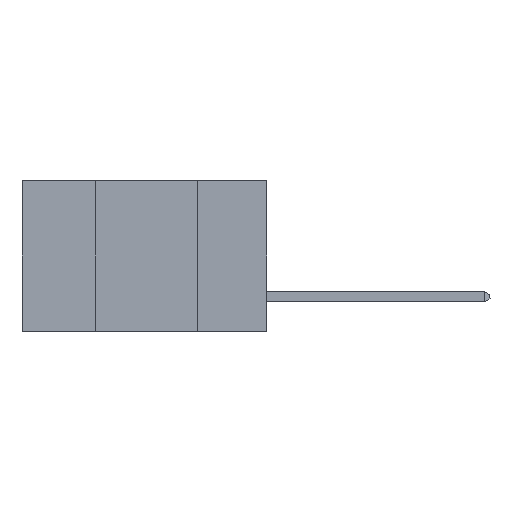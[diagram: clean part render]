
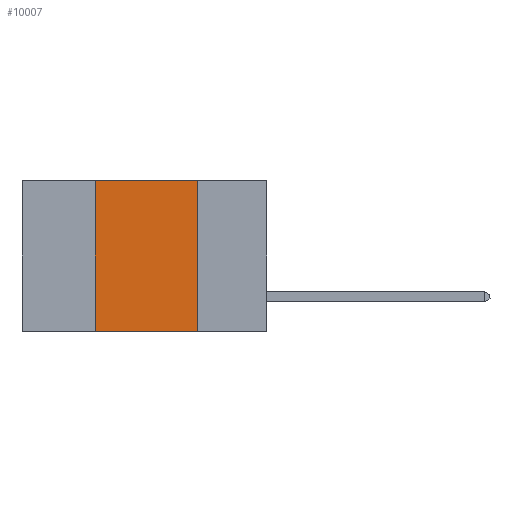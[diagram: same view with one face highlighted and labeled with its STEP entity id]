
A CAD part, left-side view. The second image highlights one B-rep face of the part: STEP entity #10007.
In plain terms, the highlighted planar face has unit normal (-1, 0, 0).
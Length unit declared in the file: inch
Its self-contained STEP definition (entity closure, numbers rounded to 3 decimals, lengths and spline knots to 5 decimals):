
#1058 = CARTESIAN_POINT ( 'NONE',  ( 0., 0.6, -0.37 ) ) ;
#1328 = VERTEX_POINT ( 'NONE', #6979 ) ;
#1591 = VECTOR ( 'NONE', #9179, 39.37008 ) ;
#1762 = PLANE ( 'NONE',  #4229 ) ;
#1782 = ORIENTED_EDGE ( 'NONE', *, *, #3634, .F. ) ;
#1858 = DIRECTION ( 'NONE',  ( 0., -1., 0. ) ) ;
#2111 = CARTESIAN_POINT ( 'NONE',  ( 0., 0.42, 0. ) ) ;
#2675 = ORIENTED_EDGE ( 'NONE', *, *, #8007, .F. ) ;
#3634 = EDGE_CURVE ( 'NONE', #5298, #1328, #10119, .T. ) ;
#3659 = VECTOR ( 'NONE', #4127, 39.37008 ) ;
#3927 = CARTESIAN_POINT ( 'NONE',  ( 0., 0.42, -0.37 ) ) ;
#4038 = ORIENTED_EDGE ( 'NONE', *, *, #4310, .F. ) ;
#4127 = DIRECTION ( 'NONE',  ( 0., 0., -1. ) ) ;
#4229 = AXIS2_PLACEMENT_3D ( 'NONE', #11930, #8880, #5949 ) ;
#4292 = VERTEX_POINT ( 'NONE', #6318 ) ;
#4310 = EDGE_CURVE ( 'NONE', #8466, #5298, #11690, .T. ) ;
#5090 = LINE ( 'NONE', #8838, #3659 ) ;
#5298 = VERTEX_POINT ( 'NONE', #12023 ) ;
#5949 = DIRECTION ( 'NONE',  ( 0., 0., -1. ) ) ;
#5994 = VECTOR ( 'NONE', #6670, 39.37008 ) ;
#6318 = CARTESIAN_POINT ( 'NONE',  ( 0., 0.17, -0.37 ) ) ;
#6670 = DIRECTION ( 'NONE',  ( 0., 0., 1. ) ) ;
#6766 = EDGE_LOOP ( 'NONE', ( #2675, #1782, #4038, #12363 ) ) ;
#6979 = CARTESIAN_POINT ( 'NONE',  ( 0., 0.17, 0. ) ) ;
#7741 = FACE_OUTER_BOUND ( 'NONE', #6766, .T. ) ;
#7770 = EDGE_CURVE ( 'NONE', #8466, #4292, #12856, .T. ) ;
#7922 = VECTOR ( 'NONE', #1858, 39.37008 ) ;
#8007 = EDGE_CURVE ( 'NONE', #1328, #4292, #5090, .T. ) ;
#8466 = VERTEX_POINT ( 'NONE', #3927 ) ;
#8838 = CARTESIAN_POINT ( 'NONE',  ( 0., 0.17, 0. ) ) ;
#8880 = DIRECTION ( 'NONE',  ( 1., 0., 0. ) ) ;
#9179 = DIRECTION ( 'NONE',  ( 0., -1., 0. ) ) ;
#10007 = ADVANCED_FACE ( 'NONE', ( #7741 ), #1762, .F. ) ;
#10119 = LINE ( 'NONE', #12155, #7922 ) ;
#11690 = LINE ( 'NONE', #2111, #5994 ) ;
#11930 = CARTESIAN_POINT ( 'NONE',  ( 0., 0.6, 0. ) ) ;
#12023 = CARTESIAN_POINT ( 'NONE',  ( 0., 0.42, 0. ) ) ;
#12155 = CARTESIAN_POINT ( 'NONE',  ( 0., 0.6, 0. ) ) ;
#12363 = ORIENTED_EDGE ( 'NONE', *, *, #7770, .T. ) ;
#12856 = LINE ( 'NONE', #1058, #1591 ) ;
